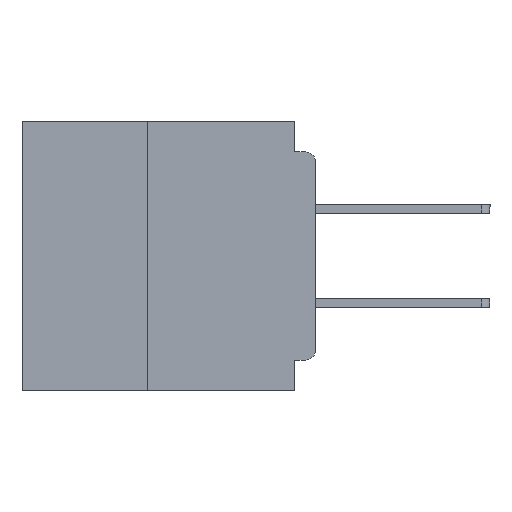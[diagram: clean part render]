
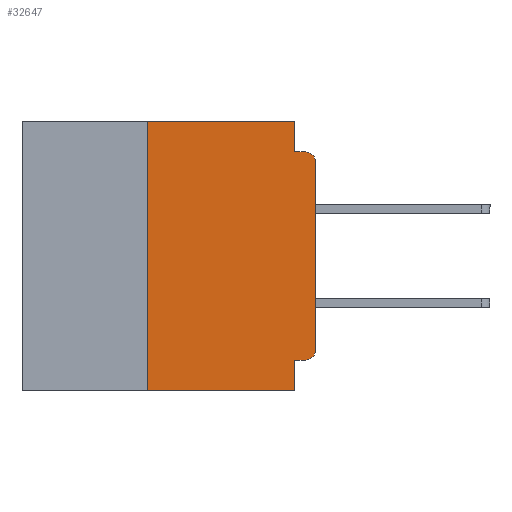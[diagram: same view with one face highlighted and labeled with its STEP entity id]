
A CAD part, left-side view. The second image highlights one B-rep face of the part: STEP entity #32647.
In plain terms, the highlighted planar face has unit normal (-1, 0, 0).
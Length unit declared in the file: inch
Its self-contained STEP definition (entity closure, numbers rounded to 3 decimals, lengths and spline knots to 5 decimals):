
#345 = ORIENTED_EDGE ( 'NONE', *, *, #44601, .T. ) ;
#825 = VECTOR ( 'NONE', #38256, 39.37008 ) ;
#829 = DIRECTION ( 'NONE',  ( 1., 0., 0. ) ) ;
#848 = VECTOR ( 'NONE', #14250, 39.37008 ) ;
#1471 = VERTEX_POINT ( 'NONE', #21678 ) ;
#2602 = CIRCLE ( 'NONE', #15597, 0.015 ) ;
#2736 = EDGE_LOOP ( 'NONE', ( #26788, #45289, #39394, #31191, #34477, #16975, #345, #28464, #10988, #39957 ) ) ;
#3629 = CARTESIAN_POINT ( 'NONE',  ( 0., 0.015, -0.355 ) ) ;
#4763 = LINE ( 'NONE', #30467, #40951 ) ;
#4969 = VERTEX_POINT ( 'NONE', #21707 ) ;
#5217 = CARTESIAN_POINT ( 'NONE',  ( 0., 0.031, -0.355 ) ) ;
#5303 = LINE ( 'NONE', #21947, #41470 ) ;
#5549 = EDGE_CURVE ( 'NONE', #23744, #4969, #20680, .T. ) ;
#5867 = FACE_OUTER_BOUND ( 'NONE', #2736, .T. ) ;
#6244 = DIRECTION ( 'NONE',  ( 0., 0., -1. ) ) ;
#7604 = LINE ( 'NONE', #26288, #43684 ) ;
#8082 = CARTESIAN_POINT ( 'NONE',  ( 0., 0.015, -0.06 ) ) ;
#8313 = CARTESIAN_POINT ( 'NONE',  ( 0., 0.015, -0.045 ) ) ;
#9551 = CARTESIAN_POINT ( 'NONE',  ( 0., 0.015, -0.34 ) ) ;
#9710 = LINE ( 'NONE', #16941, #27200 ) ;
#10988 = ORIENTED_EDGE ( 'NONE', *, *, #25156, .F. ) ;
#11646 = DIRECTION ( 'NONE',  ( 0., 0., -1. ) ) ;
#13080 = DIRECTION ( 'NONE',  ( 0., 0., -1. ) ) ;
#14250 = DIRECTION ( 'NONE',  ( 0., 0., 1. ) ) ;
#15292 = CARTESIAN_POINT ( 'NONE',  ( 0., 0.031, 0. ) ) ;
#15430 = CARTESIAN_POINT ( 'NONE',  ( 0., 0., -0.06 ) ) ;
#15597 = AXIS2_PLACEMENT_3D ( 'NONE', #9551, #34006, #13080 ) ;
#15711 = VECTOR ( 'NONE', #20546, 39.37008 ) ;
#16941 = CARTESIAN_POINT ( 'NONE',  ( 0., 0., -0.045 ) ) ;
#16975 = ORIENTED_EDGE ( 'NONE', *, *, #5549, .F. ) ;
#18158 = VERTEX_POINT ( 'NONE', #15292 ) ;
#18465 = PLANE ( 'NONE',  #40587 ) ;
#19585 = VECTOR ( 'NONE', #6244, 39.37008 ) ;
#20299 = EDGE_CURVE ( 'NONE', #27413, #43920, #24806, .T. ) ;
#20546 = DIRECTION ( 'NONE',  ( 0., 0., -1. ) ) ;
#20680 = LINE ( 'NONE', #35154, #848 ) ;
#20702 = EDGE_CURVE ( 'NONE', #18158, #32212, #24920, .T. ) ;
#20826 = VERTEX_POINT ( 'NONE', #3629 ) ;
#21678 = CARTESIAN_POINT ( 'NONE',  ( 0., 0., -0.34 ) ) ;
#21707 = CARTESIAN_POINT ( 'NONE',  ( 0., 0.25, 0. ) ) ;
#21947 = CARTESIAN_POINT ( 'NONE',  ( 0., 0.437, 0. ) ) ;
#23744 = VERTEX_POINT ( 'NONE', #28570 ) ;
#24595 = EDGE_CURVE ( 'NONE', #20826, #1471, #2602, .T. ) ;
#24806 = CIRCLE ( 'NONE', #26236, 0.015 ) ;
#24888 = VERTEX_POINT ( 'NONE', #38875 ) ;
#24920 = LINE ( 'NONE', #34514, #15711 ) ;
#25156 = EDGE_CURVE ( 'NONE', #20826, #45128, #7604, .T. ) ;
#25463 = DIRECTION ( 'NONE',  ( 0., 0., -1. ) ) ;
#25666 = EDGE_CURVE ( 'NONE', #4969, #18158, #5303, .T. ) ;
#26236 = AXIS2_PLACEMENT_3D ( 'NONE', #8082, #32580, #11646 ) ;
#26288 = CARTESIAN_POINT ( 'NONE',  ( 0., 0., -0.355 ) ) ;
#26788 = ORIENTED_EDGE ( 'NONE', *, *, #38279, .T. ) ;
#27083 = EDGE_CURVE ( 'NONE', #32212, #43920, #9710, .T. ) ;
#27200 = VECTOR ( 'NONE', #30852, 39.37008 ) ;
#27413 = VERTEX_POINT ( 'NONE', #15430 ) ;
#28464 = ORIENTED_EDGE ( 'NONE', *, *, #38201, .F. ) ;
#28570 = CARTESIAN_POINT ( 'NONE',  ( 0., 0.25, -0.4 ) ) ;
#28940 = LINE ( 'NONE', #30792, #19585 ) ;
#29852 = DIRECTION ( 'NONE',  ( 0., 1., 0. ) ) ;
#30467 = CARTESIAN_POINT ( 'NONE',  ( 0., 0.437, -0.4 ) ) ;
#30792 = CARTESIAN_POINT ( 'NONE',  ( 0., 0.031, -0.4 ) ) ;
#30852 = DIRECTION ( 'NONE',  ( 0., -1., 0. ) ) ;
#31191 = ORIENTED_EDGE ( 'NONE', *, *, #20702, .F. ) ;
#32212 = VERTEX_POINT ( 'NONE', #36524 ) ;
#32580 = DIRECTION ( 'NONE',  ( -1., 0., 0. ) ) ;
#32647 = ADVANCED_FACE ( 'NONE', ( #5867 ), #18465, .F. ) ;
#33961 = DIRECTION ( 'NONE',  ( 0., -1., 0. ) ) ;
#34006 = DIRECTION ( 'NONE',  ( -1., 0., 0. ) ) ;
#34477 = ORIENTED_EDGE ( 'NONE', *, *, #25666, .F. ) ;
#34514 = CARTESIAN_POINT ( 'NONE',  ( 0., 0.031, 0. ) ) ;
#34934 = LINE ( 'NONE', #45189, #825 ) ;
#35154 = CARTESIAN_POINT ( 'NONE',  ( 0., 0.25, -0.4 ) ) ;
#36524 = CARTESIAN_POINT ( 'NONE',  ( 0., 0.031, -0.045 ) ) ;
#38201 = EDGE_CURVE ( 'NONE', #45128, #24888, #28940, .T. ) ;
#38256 = DIRECTION ( 'NONE',  ( 0., 0., 1. ) ) ;
#38279 = EDGE_CURVE ( 'NONE', #1471, #27413, #34934, .T. ) ;
#38875 = CARTESIAN_POINT ( 'NONE',  ( 0., 0.031, -0.4 ) ) ;
#39394 = ORIENTED_EDGE ( 'NONE', *, *, #27083, .F. ) ;
#39957 = ORIENTED_EDGE ( 'NONE', *, *, #24595, .T. ) ;
#40587 = AXIS2_PLACEMENT_3D ( 'NONE', #42864, #829, #25463 ) ;
#40951 = VECTOR ( 'NONE', #33961, 39.37008 ) ;
#41470 = VECTOR ( 'NONE', #42886, 39.37008 ) ;
#42864 = CARTESIAN_POINT ( 'NONE',  ( 0., 0.437, 0. ) ) ;
#42886 = DIRECTION ( 'NONE',  ( 0., -1., 0. ) ) ;
#43684 = VECTOR ( 'NONE', #29852, 39.37008 ) ;
#43920 = VERTEX_POINT ( 'NONE', #8313 ) ;
#44601 = EDGE_CURVE ( 'NONE', #23744, #24888, #4763, .T. ) ;
#45128 = VERTEX_POINT ( 'NONE', #5217 ) ;
#45189 = CARTESIAN_POINT ( 'NONE',  ( 0., 0., 0. ) ) ;
#45289 = ORIENTED_EDGE ( 'NONE', *, *, #20299, .T. ) ;
